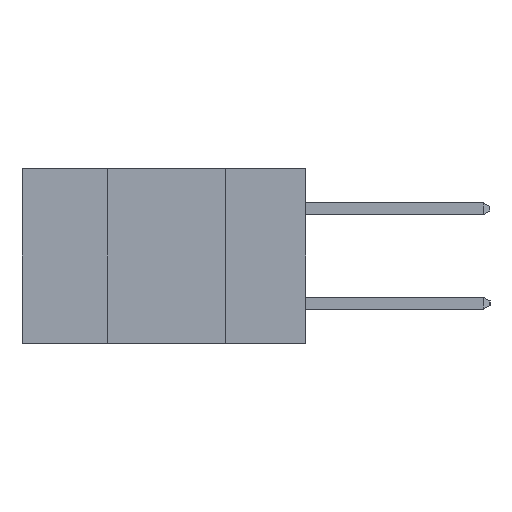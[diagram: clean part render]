
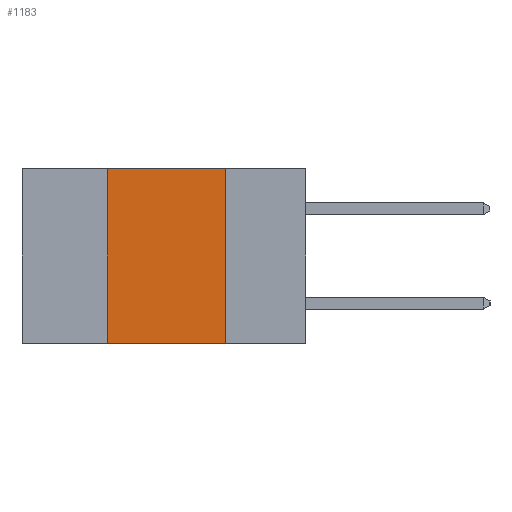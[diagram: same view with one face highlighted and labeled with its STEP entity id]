
A CAD part, left-side view. The second image highlights one B-rep face of the part: STEP entity #1183.
In plain terms, the highlighted planar face has unit normal (-1, 0, 0).
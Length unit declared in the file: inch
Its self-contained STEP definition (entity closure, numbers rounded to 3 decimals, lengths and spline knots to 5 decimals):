
#191 = DIRECTION ( 'NONE',  ( 0., 0., 1. ) ) ;
#724 = DIRECTION ( 'NONE',  ( 1., 0., 0. ) ) ;
#1030 = CARTESIAN_POINT ( 'NONE',  ( 0., 0.42, -0.37 ) ) ;
#1036 = DIRECTION ( 'NONE',  ( 0., -1., 0. ) ) ;
#1183 = ADVANCED_FACE ( 'NONE', ( #1208 ), #10224, .F. ) ;
#1208 = FACE_OUTER_BOUND ( 'NONE', #4822, .T. ) ;
#1251 = VERTEX_POINT ( 'NONE', #7398 ) ;
#1427 = EDGE_CURVE ( 'NONE', #6999, #5855, #5686, .T. ) ;
#2024 = ORIENTED_EDGE ( 'NONE', *, *, #6619, .T. ) ;
#2096 = CARTESIAN_POINT ( 'NONE',  ( 0., 0.17, -0.37 ) ) ;
#3477 = VECTOR ( 'NONE', #191, 39.37008 ) ;
#3680 = VERTEX_POINT ( 'NONE', #7586 ) ;
#3766 = LINE ( 'NONE', #10215, #7734 ) ;
#4415 = CARTESIAN_POINT ( 'NONE',  ( 0., 0.6, -0.37 ) ) ;
#4810 = CARTESIAN_POINT ( 'NONE',  ( 0., 0.42, -0.37 ) ) ;
#4822 = EDGE_LOOP ( 'NONE', ( #7705, #7932, #8169, #2024 ) ) ;
#4826 = EDGE_CURVE ( 'NONE', #5855, #1251, #3766, .T. ) ;
#4957 = DIRECTION ( 'NONE',  ( 0., -1., 0. ) ) ;
#5686 = LINE ( 'NONE', #1030, #3477 ) ;
#5855 = VERTEX_POINT ( 'NONE', #6916 ) ;
#6178 = VECTOR ( 'NONE', #1036, 39.37008 ) ;
#6202 = DIRECTION ( 'NONE',  ( 0., 0., -1. ) ) ;
#6553 = DIRECTION ( 'NONE',  ( 0., 0., -1. ) ) ;
#6619 = EDGE_CURVE ( 'NONE', #6999, #3680, #7606, .T. ) ;
#6916 = CARTESIAN_POINT ( 'NONE',  ( 0., 0.42, 0. ) ) ;
#6978 = VECTOR ( 'NONE', #6202, 39.37008 ) ;
#6999 = VERTEX_POINT ( 'NONE', #4810 ) ;
#7219 = LINE ( 'NONE', #2096, #6978 ) ;
#7398 = CARTESIAN_POINT ( 'NONE',  ( 0., 0.17, 0. ) ) ;
#7586 = CARTESIAN_POINT ( 'NONE',  ( 0., 0.17, -0.37 ) ) ;
#7606 = LINE ( 'NONE', #4415, #6178 ) ;
#7705 = ORIENTED_EDGE ( 'NONE', *, *, #7756, .F. ) ;
#7734 = VECTOR ( 'NONE', #4957, 39.37008 ) ;
#7756 = EDGE_CURVE ( 'NONE', #1251, #3680, #7219, .T. ) ;
#7932 = ORIENTED_EDGE ( 'NONE', *, *, #4826, .F. ) ;
#8169 = ORIENTED_EDGE ( 'NONE', *, *, #1427, .F. ) ;
#8779 = CARTESIAN_POINT ( 'NONE',  ( 0., 0.6, 0. ) ) ;
#9590 = AXIS2_PLACEMENT_3D ( 'NONE', #8779, #724, #6553 ) ;
#10215 = CARTESIAN_POINT ( 'NONE',  ( 0., 0.6, 0. ) ) ;
#10224 = PLANE ( 'NONE',  #9590 ) ;
